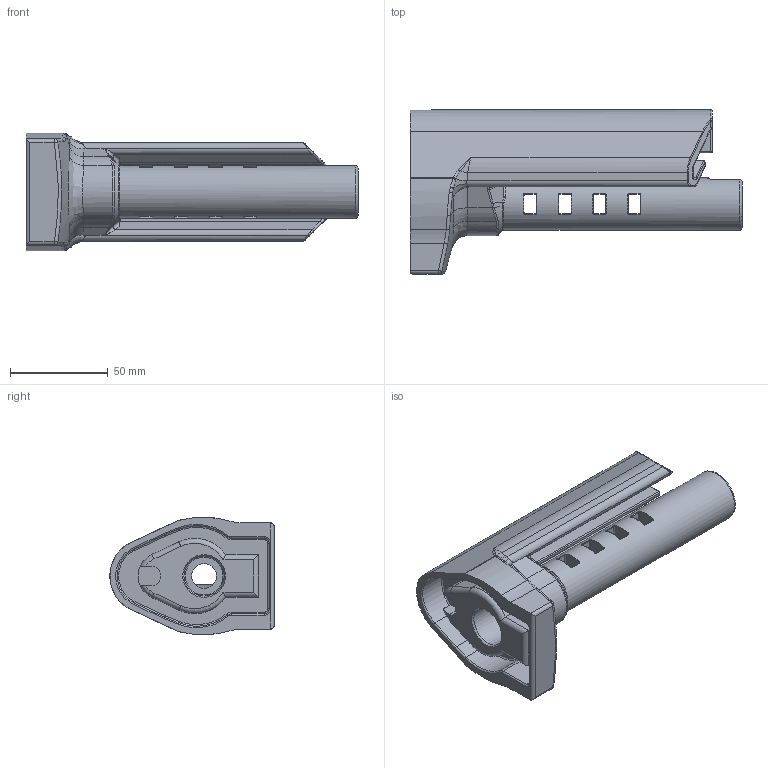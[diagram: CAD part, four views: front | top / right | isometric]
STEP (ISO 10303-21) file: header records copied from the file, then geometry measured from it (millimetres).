
FILE_DESCRIPTION(/* description */ (''),/* implementation_level */ '2;1');
FILE_NAME(/* name */ 'Mount-Cheekrest V2.stp',/* time_stamp */ '2021-12-02T15:02:56-06:00',/* author */ ('johne'),/* organization */ (''),/* preprocessor_version */ 'ST-DEVELOPER v18.1',/* originating_system */ 'Autodesk Inventor 2020',/* authorisation */ '');
FILE_SCHEMA (('AUTOMOTIVE_DESIGN { 1 0 10303 214 3 1 1 }'));
Length unit declared in the file: inch
Products named in the file (1): Pho_Spuhr_assembly - Copy
Bounding box: 170.18 x 84.15 x 60.19 mm (x, y, z)
Volume: 213247.2 mm3; surface area: 72875.8 mm2
Topology: 1 solids, 1 shells, 452 faces, 1124 edges, 655 vertices
Faces by surface type: cylinder 178, bspline 106, plane 95, torus 64, sphere 6, cone 3
Full cylindrical faces by diameter (mm): 2.75 x1, 12.725 x1, 20.599 x1, 26.924 x1
Entity records: 16894 total; most frequent: CARTESIAN_POINT 6572, ORIENTED_EDGE 2224, DIRECTION 2086, EDGE_CURVE 1112, AXIS2_PLACEMENT_3D 841, VERTEX_POINT 655, EDGE_LOOP 465, FACE_OUTER_BOUND 452
